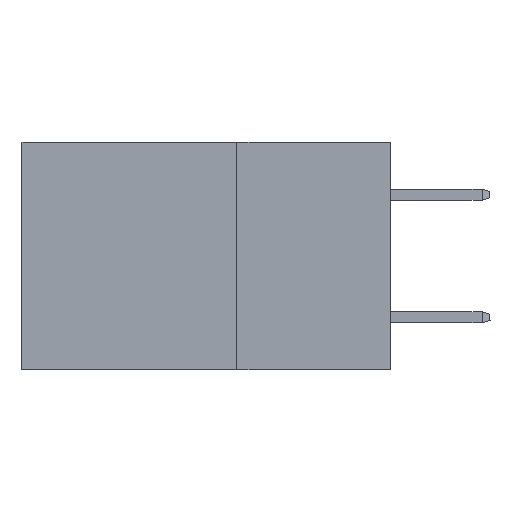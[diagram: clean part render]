
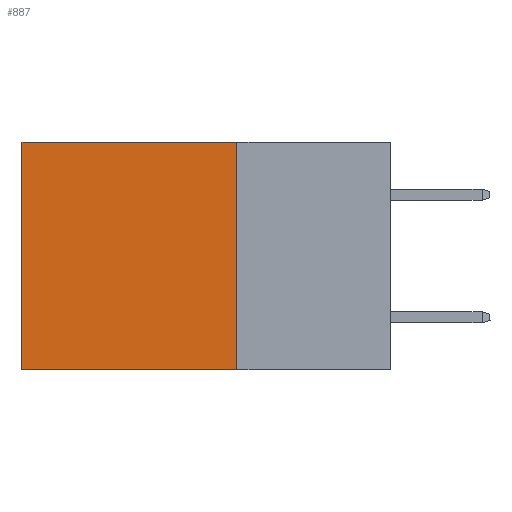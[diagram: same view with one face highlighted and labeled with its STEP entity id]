
A CAD part, left-side view. The second image highlights one B-rep face of the part: STEP entity #887.
In plain terms, the highlighted planar face has unit normal (-1, 0, 0).
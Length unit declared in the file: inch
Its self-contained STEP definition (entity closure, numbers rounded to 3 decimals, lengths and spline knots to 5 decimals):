
#283 = CARTESIAN_POINT ( 'NONE',  ( 0.2875, 0.6, -0.37 ) ) ;
#492 = EDGE_CURVE ( 'NONE', #23004, #17765, #16110, .T. ) ;
#887 = ADVANCED_FACE ( 'NONE', ( #4668 ), #12685, .F. ) ;
#960 = AXIS2_PLACEMENT_3D ( 'NONE', #6996, #9009, #8945 ) ;
#1790 = CARTESIAN_POINT ( 'NONE',  ( 0.2875, 0.25, -0.37 ) ) ;
#2284 = CARTESIAN_POINT ( 'NONE',  ( 0.2875, 0.6, 0. ) ) ;
#2812 = DIRECTION ( 'NONE',  ( 0., 1., 0. ) ) ;
#3634 = VECTOR ( 'NONE', #14132, 39.37008 ) ;
#3652 = VECTOR ( 'NONE', #18310, 39.37008 ) ;
#4508 = DIRECTION ( 'NONE',  ( 0., 1., 0. ) ) ;
#4668 = FACE_OUTER_BOUND ( 'NONE', #12619, .T. ) ;
#5587 = ORIENTED_EDGE ( 'NONE', *, *, #492, .T. ) ;
#6092 = VERTEX_POINT ( 'NONE', #283 ) ;
#6649 = VECTOR ( 'NONE', #4508, 39.37008 ) ;
#6827 = ORIENTED_EDGE ( 'NONE', *, *, #12761, .T. ) ;
#6996 = CARTESIAN_POINT ( 'NONE',  ( 0.2875, 0.25, 0. ) ) ;
#7721 = ORIENTED_EDGE ( 'NONE', *, *, #14177, .F. ) ;
#8945 = DIRECTION ( 'NONE',  ( 0., 0., -1. ) ) ;
#9009 = DIRECTION ( 'NONE',  ( 1., 0., 0. ) ) ;
#9428 = ORIENTED_EDGE ( 'NONE', *, *, #13194, .F. ) ;
#9827 = CARTESIAN_POINT ( 'NONE',  ( 0.2875, 0.25, 0. ) ) ;
#10543 = CARTESIAN_POINT ( 'NONE',  ( 0.2875, 0.25, 0. ) ) ;
#11720 = LINE ( 'NONE', #22414, #15893 ) ;
#12619 = EDGE_LOOP ( 'NONE', ( #6827, #7721, #9428, #5587 ) ) ;
#12685 = PLANE ( 'NONE',  #960 ) ;
#12761 = EDGE_CURVE ( 'NONE', #17765, #6092, #22655, .T. ) ;
#13194 = EDGE_CURVE ( 'NONE', #23004, #17360, #22630, .T. ) ;
#14132 = DIRECTION ( 'NONE',  ( 0., 0., -1. ) ) ;
#14177 = EDGE_CURVE ( 'NONE', #17360, #6092, #11720, .T. ) ;
#15893 = VECTOR ( 'NONE', #2812, 39.37008 ) ;
#16110 = LINE ( 'NONE', #21386, #6649 ) ;
#17360 = VERTEX_POINT ( 'NONE', #1790 ) ;
#17765 = VERTEX_POINT ( 'NONE', #22554 ) ;
#18310 = DIRECTION ( 'NONE',  ( 0., 0., -1. ) ) ;
#21386 = CARTESIAN_POINT ( 'NONE',  ( 0.2875, 0.25, 0. ) ) ;
#22414 = CARTESIAN_POINT ( 'NONE',  ( 0.2875, 0.25, -0.37 ) ) ;
#22554 = CARTESIAN_POINT ( 'NONE',  ( 0.2875, 0.6, 0. ) ) ;
#22630 = LINE ( 'NONE', #10543, #3634 ) ;
#22655 = LINE ( 'NONE', #2284, #3652 ) ;
#23004 = VERTEX_POINT ( 'NONE', #9827 ) ;
